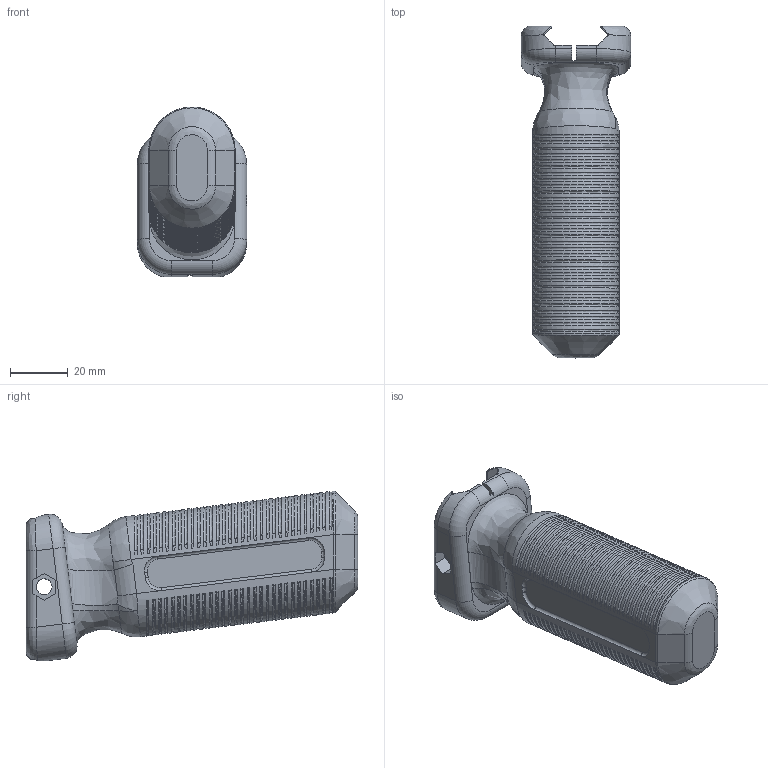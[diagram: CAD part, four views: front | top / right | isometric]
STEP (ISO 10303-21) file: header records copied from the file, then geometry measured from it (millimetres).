
FILE_DESCRIPTION(/* description */ (''),/* implementation_level */ '2;1');
FILE_NAME(/* name */ 'foregrip-picc-v2-freeman1337.step',/* time_stamp */ '2021-04-06T11:59:39-07:00',/* author */ (''),/* organization */ (''),/* preprocessor_version */ 'ST-DEVELOPER v18.1',/* originating_system */ 'Autodesk Translation Framework v9.10.0.1330',/* authorisation */ '');
FILE_SCHEMA (('AUTOMOTIVE_DESIGN { 1 0 10303 214 3 1 1 }'));
Length unit declared in the file: millimetre
Products named in the file (1): Foregrip-picc-complete-v2
Bounding box: 38 x 115.14 x 58.94 mm (x, y, z)
Volume: 114408.2 mm3; surface area: 19076 mm2
Topology: 1 solids, 1 shells, 534 faces, 1366 edges, 835 vertices
Faces by surface type: cylinder 227, bspline 190, plane 101, torus 16
Full cylindrical faces by diameter (mm): 5.5 x2, 9.75 x1
Entity records: 29555 total; most frequent: CARTESIAN_POINT 18824, ORIENTED_EDGE 2612, DIRECTION 1457, EDGE_CURVE 1306, VERTEX_POINT 835, B_SPLINE_CURVE_WITH_KNOTS 734, EDGE_LOOP 599, AXIS2_PLACEMENT_3D 540
